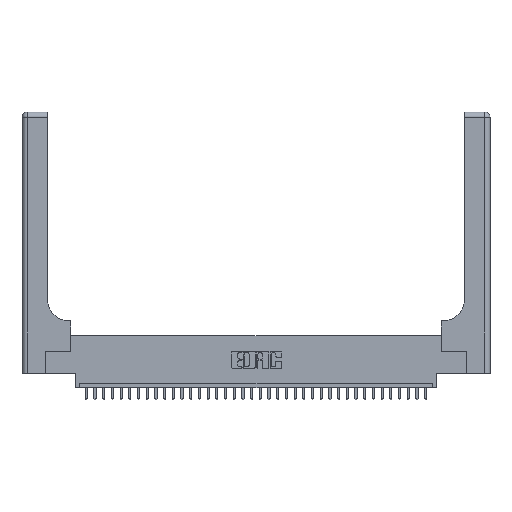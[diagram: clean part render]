
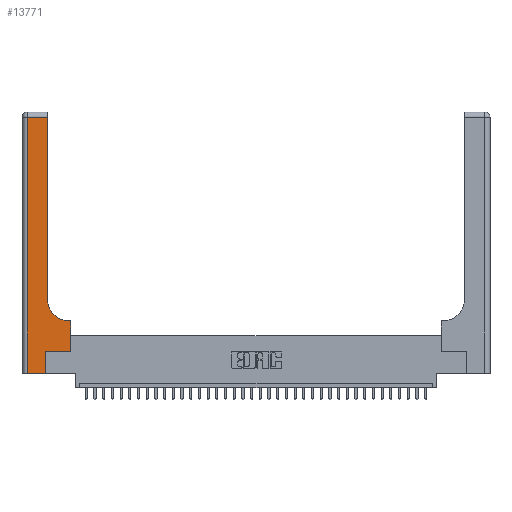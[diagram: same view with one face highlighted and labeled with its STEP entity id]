
A CAD part, top view. The second image highlights one B-rep face of the part: STEP entity #13771.
In plain terms, the highlighted planar face has unit normal (0, 0, 1).
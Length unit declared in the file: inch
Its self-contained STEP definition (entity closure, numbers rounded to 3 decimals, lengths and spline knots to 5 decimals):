
#1029 = VERTEX_POINT ( 'NONE', #23709 ) ;
#1173 = ORIENTED_EDGE ( 'NONE', *, *, #18513, .T. ) ;
#1794 = DIRECTION ( 'NONE',  ( -1., 0., 0. ) ) ;
#2268 = ORIENTED_EDGE ( 'NONE', *, *, #16534, .T. ) ;
#3299 = VECTOR ( 'NONE', #24132, 39.37008 ) ;
#3543 = DIRECTION ( 'NONE',  ( 1., 0., 0. ) ) ;
#3630 = DIRECTION ( 'NONE',  ( 1., 0., 0. ) ) ;
#4059 = CARTESIAN_POINT ( 'NONE',  ( 0.2915, 0.6, 0.37 ) ) ;
#4343 = DIRECTION ( 'NONE',  ( 0., 0., -1. ) ) ;
#4599 = CARTESIAN_POINT ( 'NONE',  ( 0., 3., 0.37 ) ) ;
#4731 = PLANE ( 'NONE',  #12864 ) ;
#5384 = CARTESIAN_POINT ( 'NONE',  ( 0.269, 0.25, 0.37 ) ) ;
#5893 = EDGE_CURVE ( 'NONE', #14082, #23223, #31084, .T. ) ;
#6392 = VECTOR ( 'NONE', #22370, 39.37008 ) ;
#7089 = ORIENTED_EDGE ( 'NONE', *, *, #5893, .T. ) ;
#7512 = CARTESIAN_POINT ( 'NONE',  ( 0.2915, 3., 0.37 ) ) ;
#7536 = LINE ( 'NONE', #11069, #26905 ) ;
#7637 = DIRECTION ( 'NONE',  ( 0., 1., 0. ) ) ;
#9306 = FACE_OUTER_BOUND ( 'NONE', #9746, .T. ) ;
#9581 = VECTOR ( 'NONE', #16450, 39.37008 ) ;
#9746 = EDGE_LOOP ( 'NONE', ( #28057, #7089, #26111, #1173, #18968, #32077, #33633, #20697, #2268 ) ) ;
#10438 = VERTEX_POINT ( 'NONE', #14133 ) ;
#10490 = DIRECTION ( 'NONE',  ( 1., 0., 0. ) ) ;
#10791 = VECTOR ( 'NONE', #18032, 39.37008 ) ;
#10824 = EDGE_CURVE ( 'NONE', #24534, #14082, #21588, .T. ) ;
#11069 = CARTESIAN_POINT ( 'NONE',  ( 0., 0., 0.37 ) ) ;
#12521 = CARTESIAN_POINT ( 'NONE',  ( 0.269, 0., 0.37 ) ) ;
#12628 = VECTOR ( 'NONE', #3543, 39.37008 ) ;
#12785 = CARTESIAN_POINT ( 'NONE',  ( 0., 2.94, 0.37 ) ) ;
#12864 = AXIS2_PLACEMENT_3D ( 'NONE', #4599, #4343, #15840 ) ;
#12960 = CARTESIAN_POINT ( 'NONE',  ( 0.2915, 0.85, 0.37 ) ) ;
#13327 = LINE ( 'NONE', #35376, #3299 ) ;
#13458 = VECTOR ( 'NONE', #7637, 39.37008 ) ;
#13633 = VERTEX_POINT ( 'NONE', #32497 ) ;
#13691 = VERTEX_POINT ( 'NONE', #30494 ) ;
#13771 = ADVANCED_FACE ( 'NONE', ( #9306 ), #4731, .F. ) ;
#14082 = VERTEX_POINT ( 'NONE', #35496 ) ;
#14133 = CARTESIAN_POINT ( 'NONE',  ( 0.5585, 0.6, 0.37 ) ) ;
#15723 = EDGE_CURVE ( 'NONE', #10438, #31456, #22317, .T. ) ;
#15840 = DIRECTION ( 'NONE',  ( -1., 0., 0. ) ) ;
#15893 = CARTESIAN_POINT ( 'NONE',  ( 0.5415, 0.85, 0.37 ) ) ;
#16450 = DIRECTION ( 'NONE',  ( 0., 1., 0. ) ) ;
#16534 = EDGE_CURVE ( 'NONE', #31456, #24534, #17096, .T. ) ;
#16723 = CARTESIAN_POINT ( 'NONE',  ( 0.06, 2.94, 0.37 ) ) ;
#17096 = CIRCLE ( 'NONE', #23413, 0.25 ) ;
#18032 = DIRECTION ( 'NONE',  ( -1., 0., 0. ) ) ;
#18513 = EDGE_CURVE ( 'NONE', #13691, #27560, #7536, .T. ) ;
#18968 = ORIENTED_EDGE ( 'NONE', *, *, #30777, .T. ) ;
#19616 = CARTESIAN_POINT ( 'NONE',  ( 0.269, 0., 0.37 ) ) ;
#19888 = LINE ( 'NONE', #5384, #12628 ) ;
#19954 = EDGE_CURVE ( 'NONE', #1029, #13633, #19888, .T. ) ;
#20485 = EDGE_CURVE ( 'NONE', #13633, #10438, #21609, .T. ) ;
#20697 = ORIENTED_EDGE ( 'NONE', *, *, #15723, .T. ) ;
#21262 = DIRECTION ( 'NONE',  ( 0., 0., -1. ) ) ;
#21588 = LINE ( 'NONE', #7512, #13458 ) ;
#21609 = LINE ( 'NONE', #35619, #9581 ) ;
#22317 = LINE ( 'NONE', #4059, #10791 ) ;
#22370 = DIRECTION ( 'NONE',  ( 0., 1., 0. ) ) ;
#23223 = VERTEX_POINT ( 'NONE', #16723 ) ;
#23413 = AXIS2_PLACEMENT_3D ( 'NONE', #15893, #21262, #10490 ) ;
#23709 = CARTESIAN_POINT ( 'NONE',  ( 0.269, 0.25, 0.37 ) ) ;
#24132 = DIRECTION ( 'NONE',  ( 0., -1., 0. ) ) ;
#24534 = VERTEX_POINT ( 'NONE', #12960 ) ;
#26111 = ORIENTED_EDGE ( 'NONE', *, *, #34806, .T. ) ;
#26905 = VECTOR ( 'NONE', #3630, 39.37008 ) ;
#27560 = VERTEX_POINT ( 'NONE', #12521 ) ;
#28057 = ORIENTED_EDGE ( 'NONE', *, *, #10824, .T. ) ;
#28375 = LINE ( 'NONE', #19616, #6392 ) ;
#28492 = CARTESIAN_POINT ( 'NONE',  ( 0.5415, 0.6, 0.37 ) ) ;
#30494 = CARTESIAN_POINT ( 'NONE',  ( 0.06, 0., 0.37 ) ) ;
#30777 = EDGE_CURVE ( 'NONE', #27560, #1029, #28375, .T. ) ;
#31084 = LINE ( 'NONE', #12785, #34577 ) ;
#31456 = VERTEX_POINT ( 'NONE', #28492 ) ;
#32077 = ORIENTED_EDGE ( 'NONE', *, *, #19954, .T. ) ;
#32497 = CARTESIAN_POINT ( 'NONE',  ( 0.5585, 0.25, 0.37 ) ) ;
#33633 = ORIENTED_EDGE ( 'NONE', *, *, #20485, .T. ) ;
#34577 = VECTOR ( 'NONE', #1794, 39.37008 ) ;
#34806 = EDGE_CURVE ( 'NONE', #23223, #13691, #13327, .T. ) ;
#35376 = CARTESIAN_POINT ( 'NONE',  ( 0.06, 3., 0.37 ) ) ;
#35496 = CARTESIAN_POINT ( 'NONE',  ( 0.2915, 2.94, 0.37 ) ) ;
#35619 = CARTESIAN_POINT ( 'NONE',  ( 0.5585, 0.25, 0.37 ) ) ;
